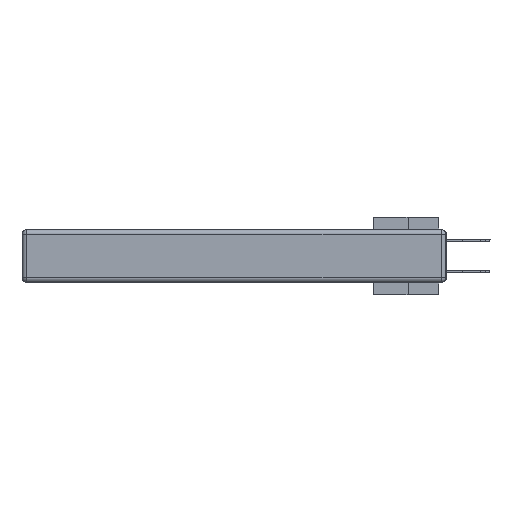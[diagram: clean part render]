
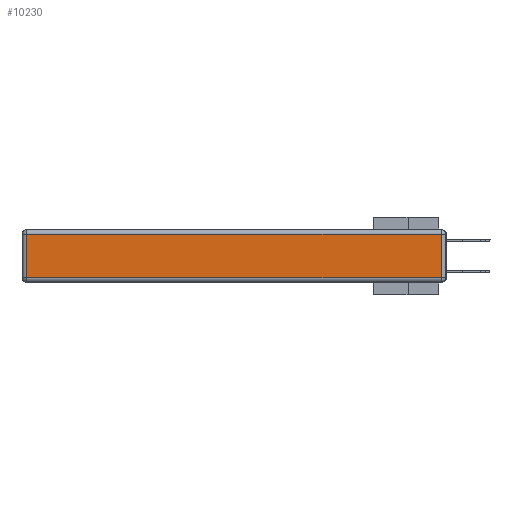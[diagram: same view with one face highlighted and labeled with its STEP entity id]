
A CAD part, left-side view. The second image highlights one B-rep face of the part: STEP entity #10230.
In plain terms, the highlighted planar face has unit normal (-1, 0, 0).
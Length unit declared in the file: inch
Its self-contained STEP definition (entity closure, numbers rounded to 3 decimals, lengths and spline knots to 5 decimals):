
#782 = ORIENTED_EDGE ( 'NONE', *, *, #23129, .T. ) ;
#890 = FACE_OUTER_BOUND ( 'NONE', #29330, .T. ) ;
#1517 = VERTEX_POINT ( 'NONE', #22455 ) ;
#3309 = ORIENTED_EDGE ( 'NONE', *, *, #3674, .T. ) ;
#3674 = EDGE_CURVE ( 'NONE', #25129, #1517, #24674, .T. ) ;
#6835 = PLANE ( 'NONE',  #34512 ) ;
#7801 = ORIENTED_EDGE ( 'NONE', *, *, #15669, .T. ) ;
#8422 = VECTOR ( 'NONE', #15451, 39.37008 ) ;
#9354 = DIRECTION ( 'NONE',  ( 0., 1., 0. ) ) ;
#10195 = LINE ( 'NONE', #23543, #8422 ) ;
#10218 = LINE ( 'NONE', #20930, #22392 ) ;
#10230 = ADVANCED_FACE ( 'NONE', ( #890 ), #6835, .T. ) ;
#10344 = LINE ( 'NONE', #31972, #33503 ) ;
#11962 = DIRECTION ( 'NONE',  ( 0., 0., 1. ) ) ;
#13219 = CARTESIAN_POINT ( 'NONE',  ( 0., 0.03, -0.313 ) ) ;
#14250 = DIRECTION ( 'NONE',  ( -1., 0., 0. ) ) ;
#15430 = DIRECTION ( 'NONE',  ( 0., 0., -1. ) ) ;
#15451 = DIRECTION ( 'NONE',  ( 0., 0., 1. ) ) ;
#15475 = DIRECTION ( 'NONE',  ( 0., -1., 0. ) ) ;
#15669 = EDGE_CURVE ( 'NONE', #29550, #25129, #10195, .T. ) ;
#17304 = ORIENTED_EDGE ( 'NONE', *, *, #22235, .T. ) ;
#17568 = VERTEX_POINT ( 'NONE', #29176 ) ;
#19702 = CARTESIAN_POINT ( 'NONE',  ( 0., 0., -0.343 ) ) ;
#20930 = CARTESIAN_POINT ( 'NONE',  ( 0., 0., -0.313 ) ) ;
#22208 = CARTESIAN_POINT ( 'NONE',  ( 0., 2.75, -0.03 ) ) ;
#22235 = EDGE_CURVE ( 'NONE', #1517, #17568, #10344, .T. ) ;
#22392 = VECTOR ( 'NONE', #15475, 39.37008 ) ;
#22455 = CARTESIAN_POINT ( 'NONE',  ( 0., 2.72, -0.03 ) ) ;
#23129 = EDGE_CURVE ( 'NONE', #17568, #29550, #10218, .T. ) ;
#23543 = CARTESIAN_POINT ( 'NONE',  ( 0., 0.03, -0.343 ) ) ;
#24674 = LINE ( 'NONE', #22208, #25942 ) ;
#25129 = VERTEX_POINT ( 'NONE', #26136 ) ;
#25942 = VECTOR ( 'NONE', #9354, 39.37008 ) ;
#26136 = CARTESIAN_POINT ( 'NONE',  ( 0., 0.03, -0.03 ) ) ;
#29176 = CARTESIAN_POINT ( 'NONE',  ( 0., 2.72, -0.313 ) ) ;
#29330 = EDGE_LOOP ( 'NONE', ( #782, #7801, #3309, #17304 ) ) ;
#29550 = VERTEX_POINT ( 'NONE', #13219 ) ;
#31972 = CARTESIAN_POINT ( 'NONE',  ( 0., 2.72, -0.343 ) ) ;
#33503 = VECTOR ( 'NONE', #15430, 39.37008 ) ;
#34512 = AXIS2_PLACEMENT_3D ( 'NONE', #19702, #14250, #11962 ) ;
